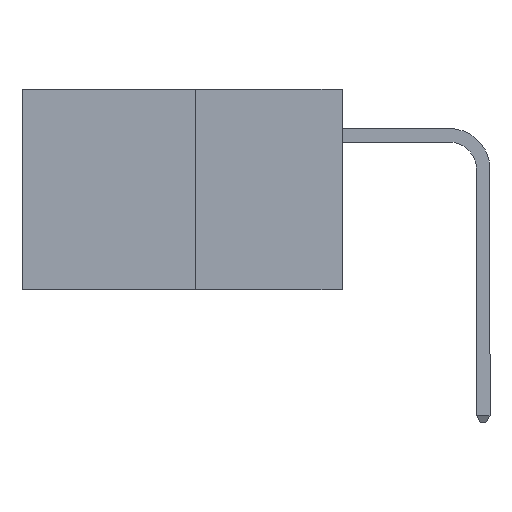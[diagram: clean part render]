
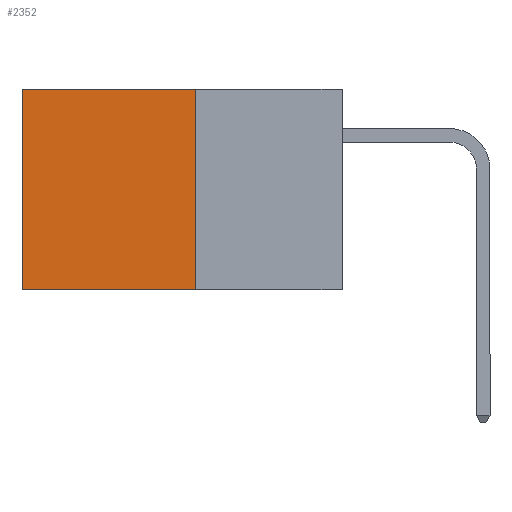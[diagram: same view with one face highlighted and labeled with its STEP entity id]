
A CAD part, left-side view. The second image highlights one B-rep face of the part: STEP entity #2352.
In plain terms, the highlighted planar face has unit normal (-1, 0, 0).
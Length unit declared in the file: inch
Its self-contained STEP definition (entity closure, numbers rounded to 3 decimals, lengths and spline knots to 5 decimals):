
#269 = DIRECTION ( 'NONE',  ( 0., 1., 0. ) ) ;
#382 = LINE ( 'NONE', #1091, #1856 ) ;
#413 = LINE ( 'NONE', #507, #3637 ) ;
#462 = VECTOR ( 'NONE', #2270, 39.37008 ) ;
#507 = CARTESIAN_POINT ( 'NONE',  ( 0.277, 0.27, 0. ) ) ;
#866 = DIRECTION ( 'NONE',  ( 1., 0., 0. ) ) ;
#1091 = CARTESIAN_POINT ( 'NONE',  ( 0.277, 0.59, -0.37 ) ) ;
#1629 = ORIENTED_EDGE ( 'NONE', *, *, #5167, .F. ) ;
#1856 = VECTOR ( 'NONE', #3010, 39.37008 ) ;
#2245 = FACE_OUTER_BOUND ( 'NONE', #2924, .T. ) ;
#2270 = DIRECTION ( 'NONE',  ( 0., 1., 0. ) ) ;
#2352 = ADVANCED_FACE ( 'NONE', ( #2245 ), #4674, .F. ) ;
#2357 = VERTEX_POINT ( 'NONE', #5827 ) ;
#2847 = CARTESIAN_POINT ( 'NONE',  ( 0.277, 0.59, 0. ) ) ;
#2924 = EDGE_LOOP ( 'NONE', ( #4806, #1629, #3556, #6765 ) ) ;
#3010 = DIRECTION ( 'NONE',  ( 0., 0., -1. ) ) ;
#3124 = EDGE_CURVE ( 'NONE', #4087, #2357, #382, .T. ) ;
#3355 = AXIS2_PLACEMENT_3D ( 'NONE', #3553, #866, #6322 ) ;
#3545 = CARTESIAN_POINT ( 'NONE',  ( 0.277, 0.27, -0.37 ) ) ;
#3553 = CARTESIAN_POINT ( 'NONE',  ( 0.277, 0.27, -0.37 ) ) ;
#3556 = ORIENTED_EDGE ( 'NONE', *, *, #5370, .F. ) ;
#3637 = VECTOR ( 'NONE', #269, 39.37008 ) ;
#3768 = VECTOR ( 'NONE', #4569, 39.37008 ) ;
#3984 = LINE ( 'NONE', #3545, #3768 ) ;
#4077 = VERTEX_POINT ( 'NONE', #7687 ) ;
#4087 = VERTEX_POINT ( 'NONE', #2847 ) ;
#4569 = DIRECTION ( 'NONE',  ( 0., 0., -1. ) ) ;
#4674 = PLANE ( 'NONE',  #3355 ) ;
#4795 = CARTESIAN_POINT ( 'NONE',  ( 0.277, 0.27, 0. ) ) ;
#4806 = ORIENTED_EDGE ( 'NONE', *, *, #3124, .T. ) ;
#5043 = VERTEX_POINT ( 'NONE', #4795 ) ;
#5167 = EDGE_CURVE ( 'NONE', #4077, #2357, #6853, .T. ) ;
#5370 = EDGE_CURVE ( 'NONE', #5043, #4077, #3984, .T. ) ;
#5441 = CARTESIAN_POINT ( 'NONE',  ( 0.277, 0.27, -0.37 ) ) ;
#5827 = CARTESIAN_POINT ( 'NONE',  ( 0.277, 0.59, -0.37 ) ) ;
#6322 = DIRECTION ( 'NONE',  ( 0., 0., -1. ) ) ;
#6765 = ORIENTED_EDGE ( 'NONE', *, *, #7055, .T. ) ;
#6853 = LINE ( 'NONE', #5441, #462 ) ;
#7055 = EDGE_CURVE ( 'NONE', #5043, #4087, #413, .T. ) ;
#7687 = CARTESIAN_POINT ( 'NONE',  ( 0.277, 0.27, -0.37 ) ) ;
